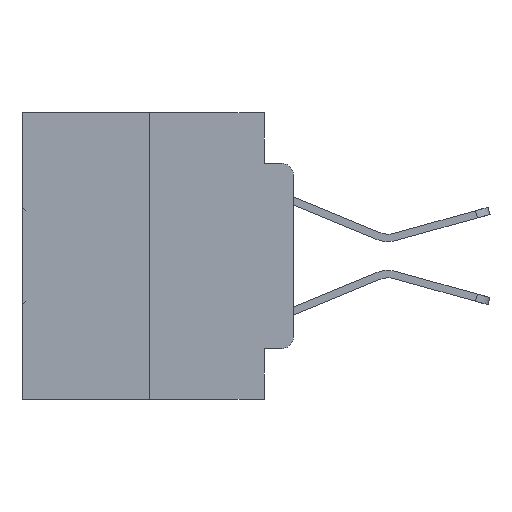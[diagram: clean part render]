
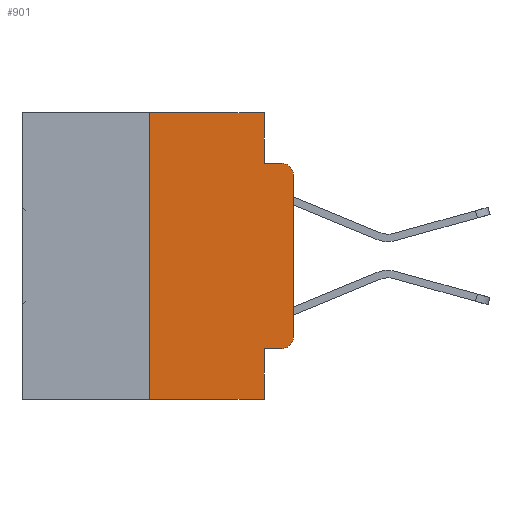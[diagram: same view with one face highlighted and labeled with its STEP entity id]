
A CAD part, left-side view. The second image highlights one B-rep face of the part: STEP entity #901.
In plain terms, the highlighted planar face has unit normal (-1, 0, 0).
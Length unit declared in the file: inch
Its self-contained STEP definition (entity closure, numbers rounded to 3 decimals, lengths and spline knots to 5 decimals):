
#49 = CARTESIAN_POINT ( 'NONE',  ( 0., 0.051, -0.0885 ) ) ;
#654 = EDGE_CURVE ( 'NONE', #25914, #19104, #2865, .T. ) ;
#901 = ADVANCED_FACE ( 'NONE', ( #14854 ), #9119, .F. ) ;
#1004 = ORIENTED_EDGE ( 'NONE', *, *, #20894, .F. ) ;
#2064 = EDGE_LOOP ( 'NONE', ( #30683, #5425, #17441, #25946, #6297, #1004, #33500, #19513, #32746, #20360 ) ) ;
#2169 = CARTESIAN_POINT ( 'NONE',  ( 0., 0.25, -0.5 ) ) ;
#2351 = DIRECTION ( 'NONE',  ( 0., -1., 0. ) ) ;
#2860 = LINE ( 'NONE', #25944, #9014 ) ;
#2865 = CIRCLE ( 'NONE', #9968, 0.02 ) ;
#2932 = CARTESIAN_POINT ( 'NONE',  ( 0., 0.051, -0.5 ) ) ;
#3351 = VERTEX_POINT ( 'NONE', #2169 ) ;
#3441 = DIRECTION ( 'NONE',  ( 0., 0., -1. ) ) ;
#3447 = LINE ( 'NONE', #33292, #9593 ) ;
#5339 = DIRECTION ( 'NONE',  ( -1., 0., 0. ) ) ;
#5425 = ORIENTED_EDGE ( 'NONE', *, *, #654, .T. ) ;
#5466 = VECTOR ( 'NONE', #9500, 39.37008 ) ;
#5812 = AXIS2_PLACEMENT_3D ( 'NONE', #11782, #14556, #12257 ) ;
#6297 = ORIENTED_EDGE ( 'NONE', *, *, #19790, .F. ) ;
#6620 = LINE ( 'NONE', #22335, #11972 ) ;
#6874 = CARTESIAN_POINT ( 'NONE',  ( 0., 0.25, 0. ) ) ;
#7039 = VECTOR ( 'NONE', #29478, 39.37008 ) ;
#7228 = DIRECTION ( 'NONE',  ( -1., 0., 0. ) ) ;
#8775 = EDGE_CURVE ( 'NONE', #14698, #15341, #6620, .T. ) ;
#9014 = VECTOR ( 'NONE', #2351, 39.37008 ) ;
#9119 = PLANE ( 'NONE',  #5812 ) ;
#9222 = DIRECTION ( 'NONE',  ( 0., 0., -1. ) ) ;
#9500 = DIRECTION ( 'NONE',  ( 0., 0., 1. ) ) ;
#9593 = VECTOR ( 'NONE', #18088, 39.37008 ) ;
#9968 = AXIS2_PLACEMENT_3D ( 'NONE', #29075, #5339, #29289 ) ;
#11782 = CARTESIAN_POINT ( 'NONE',  ( 0., 0.473, 0. ) ) ;
#11972 = VECTOR ( 'NONE', #9222, 39.37008 ) ;
#12257 = DIRECTION ( 'NONE',  ( 0., 0., -1. ) ) ;
#12864 = LINE ( 'NONE', #32096, #26716 ) ;
#14169 = AXIS2_PLACEMENT_3D ( 'NONE', #22935, #7228, #25541 ) ;
#14556 = DIRECTION ( 'NONE',  ( 1., 0., 0. ) ) ;
#14698 = VERTEX_POINT ( 'NONE', #31656 ) ;
#14854 = FACE_OUTER_BOUND ( 'NONE', #2064, .T. ) ;
#15341 = VERTEX_POINT ( 'NONE', #2932 ) ;
#16535 = VERTEX_POINT ( 'NONE', #49 ) ;
#16723 = DIRECTION ( 'NONE',  ( 0., 0., 1. ) ) ;
#16801 = CARTESIAN_POINT ( 'NONE',  ( 0., 0.051, 0. ) ) ;
#17306 = EDGE_CURVE ( 'NONE', #3351, #15341, #3447, .T. ) ;
#17441 = ORIENTED_EDGE ( 'NONE', *, *, #23923, .F. ) ;
#17672 = VERTEX_POINT ( 'NONE', #16801 ) ;
#18088 = DIRECTION ( 'NONE',  ( 0., -1., 0. ) ) ;
#19104 = VERTEX_POINT ( 'NONE', #19885 ) ;
#19132 = CARTESIAN_POINT ( 'NONE',  ( 0., 0., -0.1085 ) ) ;
#19513 = ORIENTED_EDGE ( 'NONE', *, *, #8775, .F. ) ;
#19790 = EDGE_CURVE ( 'NONE', #28746, #17672, #2860, .T. ) ;
#19885 = CARTESIAN_POINT ( 'NONE',  ( 0., 0.02, -0.0885 ) ) ;
#20084 = DIRECTION ( 'NONE',  ( 0., -1., 0. ) ) ;
#20228 = CIRCLE ( 'NONE', #14169, 0.02 ) ;
#20360 = ORIENTED_EDGE ( 'NONE', *, *, #28058, .T. ) ;
#20894 = EDGE_CURVE ( 'NONE', #3351, #28746, #26366, .T. ) ;
#21375 = VECTOR ( 'NONE', #20084, 39.37008 ) ;
#22335 = CARTESIAN_POINT ( 'NONE',  ( 0., 0.051, 0. ) ) ;
#22935 = CARTESIAN_POINT ( 'NONE',  ( 0., 0.02, -0.3915 ) ) ;
#23923 = EDGE_CURVE ( 'NONE', #16535, #19104, #29762, .T. ) ;
#23959 = CARTESIAN_POINT ( 'NONE',  ( 0., 0.02, -0.4115 ) ) ;
#24341 = CARTESIAN_POINT ( 'NONE',  ( 0., 0.051, 0. ) ) ;
#25008 = EDGE_CURVE ( 'NONE', #17672, #16535, #32834, .T. ) ;
#25541 = DIRECTION ( 'NONE',  ( 0., 0., -1. ) ) ;
#25914 = VERTEX_POINT ( 'NONE', #19132 ) ;
#25944 = CARTESIAN_POINT ( 'NONE',  ( 0., 0.473, 0. ) ) ;
#25946 = ORIENTED_EDGE ( 'NONE', *, *, #25008, .F. ) ;
#26100 = VECTOR ( 'NONE', #3441, 39.37008 ) ;
#26136 = VERTEX_POINT ( 'NONE', #27665 ) ;
#26366 = LINE ( 'NONE', #6874, #5466 ) ;
#26716 = VECTOR ( 'NONE', #16723, 39.37008 ) ;
#26964 = CARTESIAN_POINT ( 'NONE',  ( 0., 0.051, -0.4115 ) ) ;
#27665 = CARTESIAN_POINT ( 'NONE',  ( 0., 0., -0.3915 ) ) ;
#27821 = EDGE_CURVE ( 'NONE', #26136, #25914, #12864, .T. ) ;
#27854 = LINE ( 'NONE', #26964, #7039 ) ;
#28058 = EDGE_CURVE ( 'NONE', #33359, #26136, #20228, .T. ) ;
#28434 = EDGE_CURVE ( 'NONE', #14698, #33359, #27854, .T. ) ;
#28746 = VERTEX_POINT ( 'NONE', #32675 ) ;
#29075 = CARTESIAN_POINT ( 'NONE',  ( 0., 0.02, -0.1085 ) ) ;
#29289 = DIRECTION ( 'NONE',  ( 0., 0., -1. ) ) ;
#29478 = DIRECTION ( 'NONE',  ( 0., -1., 0. ) ) ;
#29762 = LINE ( 'NONE', #32840, #21375 ) ;
#30683 = ORIENTED_EDGE ( 'NONE', *, *, #27821, .T. ) ;
#31656 = CARTESIAN_POINT ( 'NONE',  ( 0., 0.051, -0.4115 ) ) ;
#32096 = CARTESIAN_POINT ( 'NONE',  ( 0., 0., 0. ) ) ;
#32675 = CARTESIAN_POINT ( 'NONE',  ( 0., 0.25, 0. ) ) ;
#32746 = ORIENTED_EDGE ( 'NONE', *, *, #28434, .T. ) ;
#32834 = LINE ( 'NONE', #24341, #26100 ) ;
#32840 = CARTESIAN_POINT ( 'NONE',  ( 0., 0.051, -0.0885 ) ) ;
#33292 = CARTESIAN_POINT ( 'NONE',  ( 0., 0.473, -0.5 ) ) ;
#33359 = VERTEX_POINT ( 'NONE', #23959 ) ;
#33500 = ORIENTED_EDGE ( 'NONE', *, *, #17306, .T. ) ;
